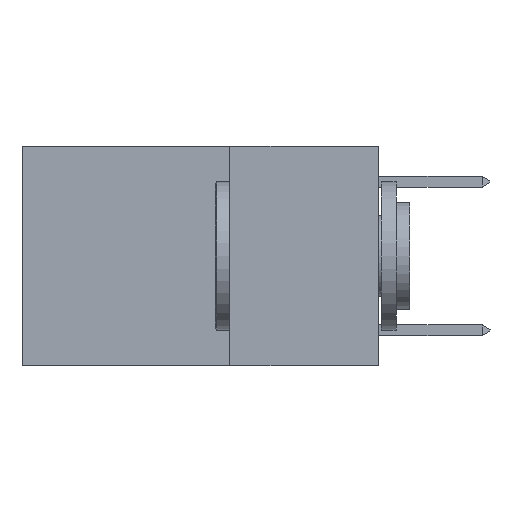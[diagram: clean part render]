
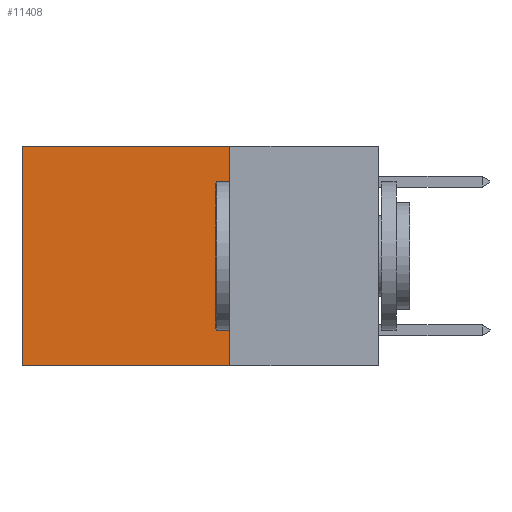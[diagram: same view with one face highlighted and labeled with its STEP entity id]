
A CAD part, left-side view. The second image highlights one B-rep face of the part: STEP entity #11408.
In plain terms, the highlighted planar face has unit normal (-1, 0, 0).
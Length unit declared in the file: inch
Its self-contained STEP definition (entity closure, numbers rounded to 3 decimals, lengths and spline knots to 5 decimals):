
#687 = VECTOR ( 'NONE', #18652, 39.37008 ) ;
#826 = LINE ( 'NONE', #18773, #687 ) ;
#1329 = DIRECTION ( 'NONE',  ( 0., 0., -1. ) ) ;
#1602 = AXIS2_PLACEMENT_3D ( 'NONE', #21388, #21145, #21017 ) ;
#1635 = DIRECTION ( 'NONE',  ( 0., 0., -1. ) ) ;
#1850 = CARTESIAN_POINT ( 'NONE',  ( 0.2625, 0.6, 0. ) ) ;
#2073 = CARTESIAN_POINT ( 'NONE',  ( 0.2625, 0.25, 0. ) ) ;
#2693 = VERTEX_POINT ( 'NONE', #5673 ) ;
#5015 = ORIENTED_EDGE ( 'NONE', *, *, #12933, .T. ) ;
#5673 = CARTESIAN_POINT ( 'NONE',  ( 0.2625, 0.25, 0. ) ) ;
#6368 = EDGE_LOOP ( 'NONE', ( #5015, #6909, #7032, #10019 ) ) ;
#6631 = DIRECTION ( 'NONE',  ( 0., 1., 0. ) ) ;
#6828 = VERTEX_POINT ( 'NONE', #16094 ) ;
#6909 = ORIENTED_EDGE ( 'NONE', *, *, #7683, .F. ) ;
#7032 = ORIENTED_EDGE ( 'NONE', *, *, #20248, .F. ) ;
#7527 = CARTESIAN_POINT ( 'NONE',  ( 0.2625, 0.25, 0. ) ) ;
#7683 = EDGE_CURVE ( 'NONE', #23824, #6828, #826, .T. ) ;
#7897 = FACE_OUTER_BOUND ( 'NONE', #6368, .T. ) ;
#7922 = VERTEX_POINT ( 'NONE', #11113 ) ;
#10019 = ORIENTED_EDGE ( 'NONE', *, *, #19409, .T. ) ;
#11113 = CARTESIAN_POINT ( 'NONE',  ( 0.2625, 0.6, 0. ) ) ;
#11408 = ADVANCED_FACE ( 'NONE', ( #7897 ), #21279, .F. ) ;
#12933 = EDGE_CURVE ( 'NONE', #7922, #6828, #13243, .T. ) ;
#12999 = VECTOR ( 'NONE', #1329, 39.37008 ) ;
#13243 = LINE ( 'NONE', #1850, #12999 ) ;
#13917 = VECTOR ( 'NONE', #1635, 39.37008 ) ;
#14132 = LINE ( 'NONE', #2073, #13917 ) ;
#16094 = CARTESIAN_POINT ( 'NONE',  ( 0.2625, 0.6, -0.37 ) ) ;
#18652 = DIRECTION ( 'NONE',  ( 0., 1., 0. ) ) ;
#18773 = CARTESIAN_POINT ( 'NONE',  ( 0.2625, 0.25, -0.37 ) ) ;
#19409 = EDGE_CURVE ( 'NONE', #2693, #7922, #19746, .T. ) ;
#19671 = VECTOR ( 'NONE', #6631, 39.37008 ) ;
#19746 = LINE ( 'NONE', #7527, #19671 ) ;
#20248 = EDGE_CURVE ( 'NONE', #2693, #23824, #14132, .T. ) ;
#21017 = DIRECTION ( 'NONE',  ( 0., 0., -1. ) ) ;
#21145 = DIRECTION ( 'NONE',  ( 1., 0., 0. ) ) ;
#21279 = PLANE ( 'NONE',  #1602 ) ;
#21388 = CARTESIAN_POINT ( 'NONE',  ( 0.2625, 0.25, 0. ) ) ;
#23298 = CARTESIAN_POINT ( 'NONE',  ( 0.2625, 0.25, -0.37 ) ) ;
#23824 = VERTEX_POINT ( 'NONE', #23298 ) ;
